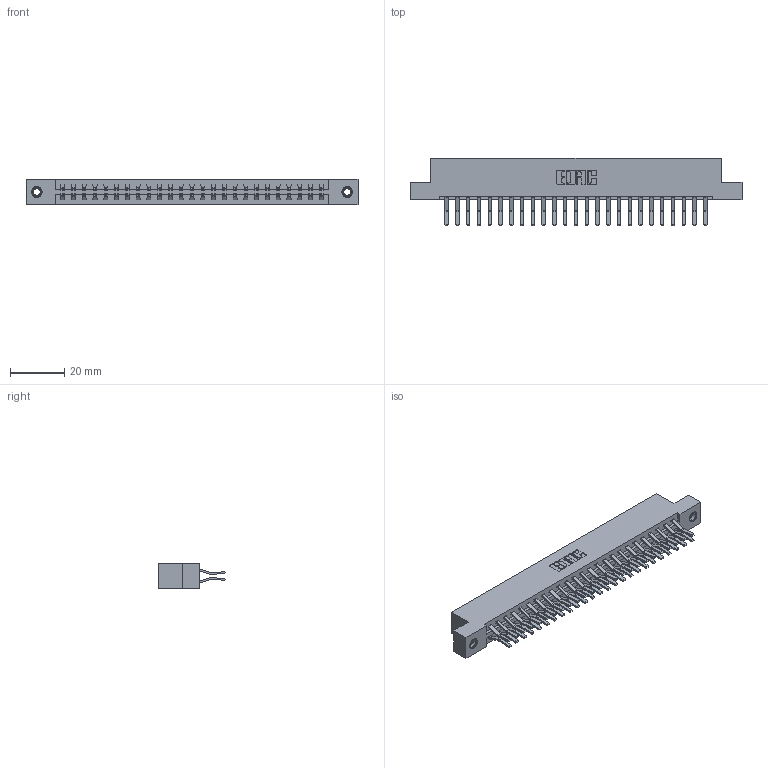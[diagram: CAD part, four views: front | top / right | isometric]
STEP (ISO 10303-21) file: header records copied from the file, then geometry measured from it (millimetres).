
FILE_DESCRIPTION (( 'STEP AP203' ), '1' );
FILE_NAME ('337-050-560-207.STEP', '2019-10-09T16:22:22', ( '' ), ( '' ), 'SwSTEP 2.0', 'SolidWorks 2016', '' );
FILE_SCHEMA (( 'CONFIG_CONTROL_DESIGN' ));
Length unit declared in the file: inch
Products named in the file (4): 337-050-560-207; 337 Part_Flush Mounting Lugs - 0.156 Dia-TI; 345-292-001_560 Tail; 345-250-001_345-250-005-103
Assembly tree (53 placements, depth 2):
  337-050-560-207
    337 Part_Flush Mounting Lugs - 0.156 Dia-TI
    345-292-001_560 Tail  x50
    345-250-001_345-250-005-103  x2
Bounding box: 122.07 x 24.78 x 9.4 mm (x, y, z)
Volume: 12952.9 mm3; surface area: 15462.6 mm2
Topology: 53 solids, 53 shells, 2974 faces, 8797 edges, 5790 vertices
Faces by surface type: plane 2002, cylinder 956, cone 12, torus 4
Entity records: 22856 total; most frequent: CARTESIAN_POINT 3845, ORIENTED_EDGE 3774, DIRECTION 3337, EDGE_CURVE 1887, VECTOR 1735, LINE 1735, VERTEX_POINT 1252, AXIS2_PLACEMENT_3D 801
